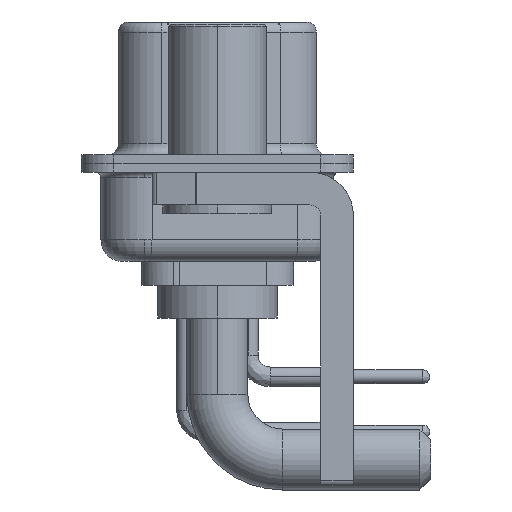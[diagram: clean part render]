
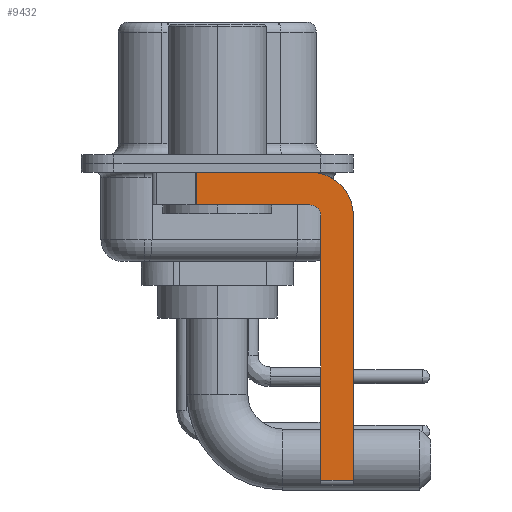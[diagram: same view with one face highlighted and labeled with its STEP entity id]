
A CAD part, left-side view. The second image highlights one B-rep face of the part: STEP entity #9432.
In plain terms, the highlighted planar face has unit normal (-1, 0, 0).
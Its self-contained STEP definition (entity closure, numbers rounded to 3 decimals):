
#1028 = CARTESIAN_POINT ( 'NONE',  ( -2.9, -4.25, -1.9 ) ) ;
#2267 = EDGE_CURVE ( 'NONE', #11700, #27676, #14378, .T. ) ;
#2326 = VECTOR ( 'NONE', #27944, 1000. ) ;
#2342 = CARTESIAN_POINT ( 'NONE',  ( -2.9, -6.25, -2.4 ) ) ;
#2441 = VERTEX_POINT ( 'NONE', #12101 ) ;
#2961 = VERTEX_POINT ( 'NONE', #8494 ) ;
#3077 = EDGE_CURVE ( 'NONE', #2961, #20703, #10220, .T. ) ;
#4161 = DIRECTION ( 'NONE',  ( -1., 0., 0. ) ) ;
#4457 = ORIENTED_EDGE ( 'NONE', *, *, #6422, .T. ) ;
#5435 = VECTOR ( 'NONE', #24118, 1000. ) ;
#5736 = AXIS2_PLACEMENT_3D ( 'NONE', #19410, #4161, #19550 ) ;
#5962 = ORIENTED_EDGE ( 'NONE', *, *, #2267, .F. ) ;
#6416 = EDGE_LOOP ( 'NONE', ( #16233, #4457, #16201, #5962, #23818, #16444, #21043, #26211 ) ) ;
#6422 = EDGE_CURVE ( 'NONE', #15662, #23563, #20771, .T. ) ;
#6534 = DIRECTION ( 'NONE',  ( 0., 0., -1. ) ) ;
#6613 = CARTESIAN_POINT ( 'NONE',  ( -2.9, -4.75, -2.4 ) ) ;
#8106 = DIRECTION ( 'NONE',  ( 0., 0., 1. ) ) ;
#8494 = CARTESIAN_POINT ( 'NONE',  ( -2.9, -4.25, -0.4 ) ) ;
#8593 = EDGE_CURVE ( 'NONE', #27676, #23563, #27081, .T. ) ;
#9432 = ADVANCED_FACE ( 'NONE', ( #16504 ), #11623, .F. ) ;
#10085 = VECTOR ( 'NONE', #12140, 1000. ) ;
#10093 = DIRECTION ( 'NONE',  ( 0., 0., -1. ) ) ;
#10186 = VECTOR ( 'NONE', #8106, 1000. ) ;
#10220 = CIRCLE ( 'NONE', #26111, 2. ) ;
#11584 = CARTESIAN_POINT ( 'NONE',  ( -2.9, -4.75, -14.8 ) ) ;
#11623 = PLANE ( 'NONE',  #21463 ) ;
#11700 = VERTEX_POINT ( 'NONE', #6613 ) ;
#12101 = CARTESIAN_POINT ( 'NONE',  ( -2.9, -4.75, -14.55 ) ) ;
#12140 = DIRECTION ( 'NONE',  ( 0., 1., 0. ) ) ;
#12165 = DIRECTION ( 'NONE',  ( 0., -1., 0. ) ) ;
#12708 = LINE ( 'NONE', #19259, #2326 ) ;
#12912 = CARTESIAN_POINT ( 'NONE',  ( -2.9, 0.978, -0.4 ) ) ;
#13042 = CARTESIAN_POINT ( 'NONE',  ( -2.9, -4.25, -2.4 ) ) ;
#13168 = VECTOR ( 'NONE', #10093, 1000. ) ;
#14218 = CARTESIAN_POINT ( 'NONE',  ( -2.9, 0.978, -1.9 ) ) ;
#14296 = VERTEX_POINT ( 'NONE', #28137 ) ;
#14378 = CIRCLE ( 'NONE', #5736, 0.5 ) ;
#15148 = CARTESIAN_POINT ( 'NONE',  ( -2.9, -6.25, -2.4 ) ) ;
#15662 = VERTEX_POINT ( 'NONE', #12912 ) ;
#16015 = DIRECTION ( 'NONE',  ( 1., 0., 0. ) ) ;
#16201 = ORIENTED_EDGE ( 'NONE', *, *, #8593, .F. ) ;
#16233 = ORIENTED_EDGE ( 'NONE', *, *, #27054, .F. ) ;
#16444 = ORIENTED_EDGE ( 'NONE', *, *, #17307, .T. ) ;
#16504 = FACE_OUTER_BOUND ( 'NONE', #6416, .T. ) ;
#17307 = EDGE_CURVE ( 'NONE', #2441, #14296, #26553, .T. ) ;
#17737 = DIRECTION ( 'NONE',  ( 0., 0., -1. ) ) ;
#17792 = EDGE_CURVE ( 'NONE', #2441, #11700, #22530, .T. ) ;
#19259 = CARTESIAN_POINT ( 'NONE',  ( -2.9, 3., -0.4 ) ) ;
#19410 = CARTESIAN_POINT ( 'NONE',  ( -2.9, -4.25, -2.4 ) ) ;
#19550 = DIRECTION ( 'NONE',  ( 0., 0., 1. ) ) ;
#20703 = VERTEX_POINT ( 'NONE', #15148 ) ;
#20707 = CARTESIAN_POINT ( 'NONE',  ( -2.9, -4.25, -14.55 ) ) ;
#20771 = LINE ( 'NONE', #14218, #13168 ) ;
#21043 = ORIENTED_EDGE ( 'NONE', *, *, #25379, .F. ) ;
#21463 = AXIS2_PLACEMENT_3D ( 'NONE', #23886, #16015, #6534 ) ;
#22349 = CARTESIAN_POINT ( 'NONE',  ( -2.9, -4.25, -1.9 ) ) ;
#22463 = CARTESIAN_POINT ( 'NONE',  ( -2.9, 0.978, -1.9 ) ) ;
#22530 = LINE ( 'NONE', #11584, #10186 ) ;
#23563 = VERTEX_POINT ( 'NONE', #22463 ) ;
#23818 = ORIENTED_EDGE ( 'NONE', *, *, #17792, .F. ) ;
#23886 = CARTESIAN_POINT ( 'NONE',  ( -2.9, -4.25, -2.4 ) ) ;
#24118 = DIRECTION ( 'NONE',  ( 0., 0., -1. ) ) ;
#24261 = LINE ( 'NONE', #2342, #5435 ) ;
#24684 = VECTOR ( 'NONE', #12165, 1000. ) ;
#25379 = EDGE_CURVE ( 'NONE', #20703, #14296, #24261, .T. ) ;
#26111 = AXIS2_PLACEMENT_3D ( 'NONE', #13042, #26274, #17737 ) ;
#26211 = ORIENTED_EDGE ( 'NONE', *, *, #3077, .F. ) ;
#26274 = DIRECTION ( 'NONE',  ( 1., 0., 0. ) ) ;
#26553 = LINE ( 'NONE', #20707, #24684 ) ;
#27054 = EDGE_CURVE ( 'NONE', #15662, #2961, #12708, .T. ) ;
#27081 = LINE ( 'NONE', #1028, #10085 ) ;
#27676 = VERTEX_POINT ( 'NONE', #22349 ) ;
#27944 = DIRECTION ( 'NONE',  ( 0., -1., 0. ) ) ;
#28137 = CARTESIAN_POINT ( 'NONE',  ( -2.9, -6.25, -14.55 ) ) ;
